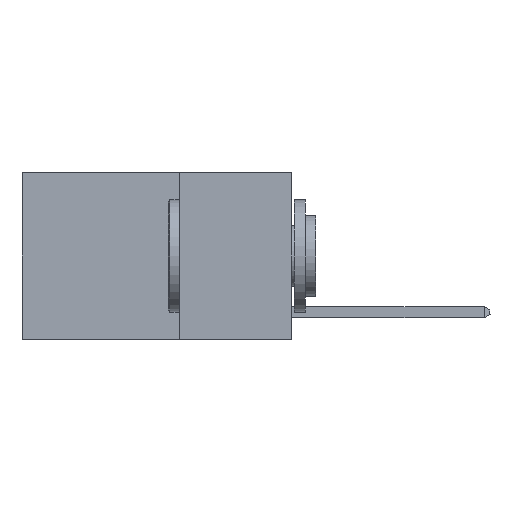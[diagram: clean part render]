
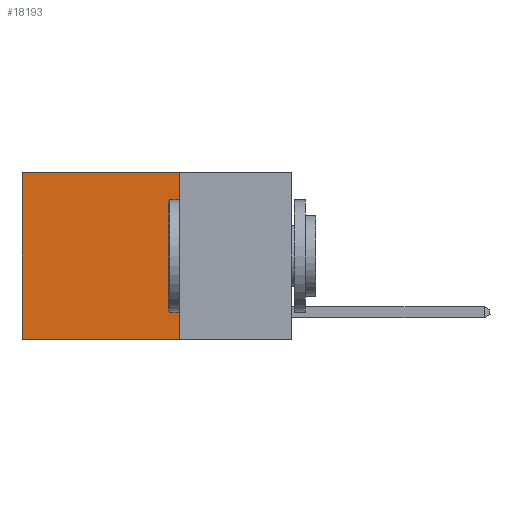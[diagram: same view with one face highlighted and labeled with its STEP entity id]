
A CAD part, left-side view. The second image highlights one B-rep face of the part: STEP entity #18193.
In plain terms, the highlighted planar face has unit normal (-1, 0, 0).
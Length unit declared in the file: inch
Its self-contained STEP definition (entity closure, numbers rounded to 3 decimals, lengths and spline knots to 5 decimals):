
#117 = CARTESIAN_POINT ( 'NONE',  ( 0.2625, 0.25, -0.37 ) ) ;
#571 = VERTEX_POINT ( 'NONE', #117 ) ;
#776 = VERTEX_POINT ( 'NONE', #11007 ) ;
#2577 = DIRECTION ( 'NONE',  ( 1., 0., 0. ) ) ;
#4716 = EDGE_CURVE ( 'NONE', #22311, #571, #15604, .T. ) ;
#4755 = CARTESIAN_POINT ( 'NONE',  ( 0.2625, 0.25, 0. ) ) ;
#4871 = CARTESIAN_POINT ( 'NONE',  ( 0.2625, 0.6, 0. ) ) ;
#6605 = CARTESIAN_POINT ( 'NONE',  ( 0.2625, 0.25, -0.37 ) ) ;
#6845 = VERTEX_POINT ( 'NONE', #13726 ) ;
#8773 = ORIENTED_EDGE ( 'NONE', *, *, #13096, .F. ) ;
#9142 = LINE ( 'NONE', #4871, #19239 ) ;
#9906 = ORIENTED_EDGE ( 'NONE', *, *, #21727, .T. ) ;
#10669 = PLANE ( 'NONE',  #15398 ) ;
#11007 = CARTESIAN_POINT ( 'NONE',  ( 0.2625, 0.6, -0.37 ) ) ;
#12615 = FACE_OUTER_BOUND ( 'NONE', #14959, .T. ) ;
#13096 = EDGE_CURVE ( 'NONE', #571, #776, #19229, .T. ) ;
#13726 = CARTESIAN_POINT ( 'NONE',  ( 0.2625, 0.6, 0. ) ) ;
#13837 = ORIENTED_EDGE ( 'NONE', *, *, #25210, .T. ) ;
#13844 = CARTESIAN_POINT ( 'NONE',  ( 0.2625, 0.25, 0. ) ) ;
#14764 = CARTESIAN_POINT ( 'NONE',  ( 0.2625, 0.25, 0. ) ) ;
#14790 = DIRECTION ( 'NONE',  ( 0., 1., 0. ) ) ;
#14959 = EDGE_LOOP ( 'NONE', ( #9906, #8773, #17769, #13837 ) ) ;
#14967 = DIRECTION ( 'NONE',  ( 0., 0., -1. ) ) ;
#15398 = AXIS2_PLACEMENT_3D ( 'NONE', #14764, #2577, #16734 ) ;
#15604 = LINE ( 'NONE', #13844, #23772 ) ;
#16734 = DIRECTION ( 'NONE',  ( 0., 0., -1. ) ) ;
#17325 = VECTOR ( 'NONE', #14790, 39.37008 ) ;
#17769 = ORIENTED_EDGE ( 'NONE', *, *, #4716, .F. ) ;
#18193 = ADVANCED_FACE ( 'NONE', ( #12615 ), #10669, .F. ) ;
#19229 = LINE ( 'NONE', #6605, #17325 ) ;
#19239 = VECTOR ( 'NONE', #14967, 39.37008 ) ;
#20973 = LINE ( 'NONE', #23467, #25697 ) ;
#21727 = EDGE_CURVE ( 'NONE', #6845, #776, #9142, .T. ) ;
#22311 = VERTEX_POINT ( 'NONE', #4755 ) ;
#23467 = CARTESIAN_POINT ( 'NONE',  ( 0.2625, 0.25, 0. ) ) ;
#23772 = VECTOR ( 'NONE', #23851, 39.37008 ) ;
#23851 = DIRECTION ( 'NONE',  ( 0., 0., -1. ) ) ;
#25210 = EDGE_CURVE ( 'NONE', #22311, #6845, #20973, .T. ) ;
#25492 = DIRECTION ( 'NONE',  ( 0., 1., 0. ) ) ;
#25697 = VECTOR ( 'NONE', #25492, 39.37008 ) ;
